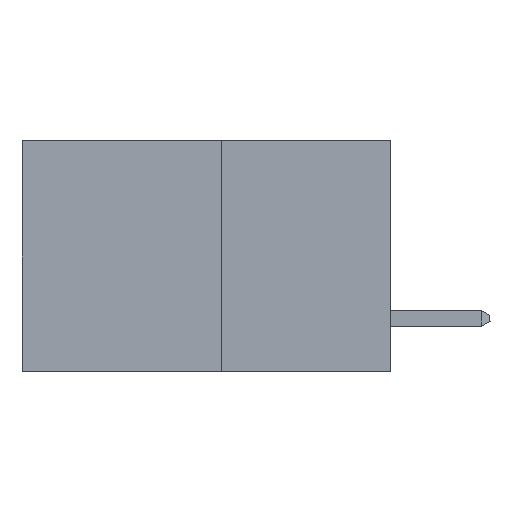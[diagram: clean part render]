
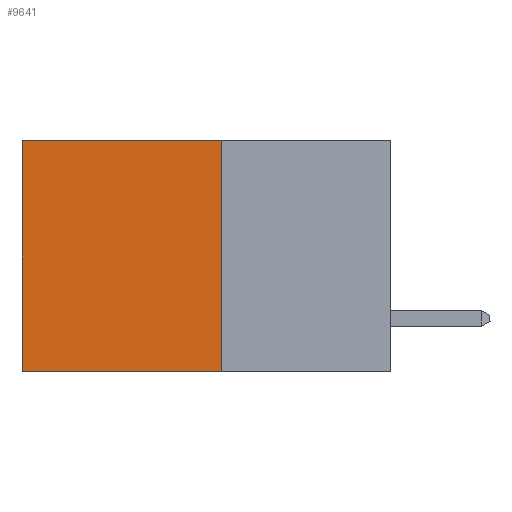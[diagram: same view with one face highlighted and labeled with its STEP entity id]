
A CAD part, left-side view. The second image highlights one B-rep face of the part: STEP entity #9641.
In plain terms, the highlighted planar face has unit normal (-1, 0, 0).
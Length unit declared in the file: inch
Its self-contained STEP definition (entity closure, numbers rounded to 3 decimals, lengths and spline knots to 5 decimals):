
#358 = AXIS2_PLACEMENT_3D ( 'NONE', #10033, #2748, #11231 ) ;
#535 = EDGE_CURVE ( 'NONE', #11754, #8531, #8015, .T. ) ;
#1074 = CARTESIAN_POINT ( 'NONE',  ( 0.277, 0.59, 0. ) ) ;
#1254 = EDGE_CURVE ( 'NONE', #7984, #7675, #7183, .T. ) ;
#1770 = LINE ( 'NONE', #3849, #7908 ) ;
#2586 = DIRECTION ( 'NONE',  ( 0., 1., 0. ) ) ;
#2630 = PLANE ( 'NONE',  #358 ) ;
#2748 = DIRECTION ( 'NONE',  ( 1., 0., 0. ) ) ;
#3657 = ORIENTED_EDGE ( 'NONE', *, *, #9433, .F. ) ;
#3849 = CARTESIAN_POINT ( 'NONE',  ( 0.277, 0.27, 0. ) ) ;
#3951 = VECTOR ( 'NONE', #7203, 39.37008 ) ;
#5088 = VECTOR ( 'NONE', #8420, 39.37008 ) ;
#5573 = ORIENTED_EDGE ( 'NONE', *, *, #535, .F. ) ;
#6667 = CARTESIAN_POINT ( 'NONE',  ( 0.277, 0.27, -0.37 ) ) ;
#7183 = LINE ( 'NONE', #7550, #3951 ) ;
#7203 = DIRECTION ( 'NONE',  ( 0., 0., -1. ) ) ;
#7550 = CARTESIAN_POINT ( 'NONE',  ( 0.277, 0.59, -0.37 ) ) ;
#7675 = VERTEX_POINT ( 'NONE', #9093 ) ;
#7908 = VECTOR ( 'NONE', #2586, 39.37008 ) ;
#7984 = VERTEX_POINT ( 'NONE', #1074 ) ;
#8015 = LINE ( 'NONE', #6667, #13996 ) ;
#8255 = LINE ( 'NONE', #10805, #5088 ) ;
#8387 = CARTESIAN_POINT ( 'NONE',  ( 0.277, 0.27, 0. ) ) ;
#8420 = DIRECTION ( 'NONE',  ( 0., 1., 0. ) ) ;
#8439 = FACE_OUTER_BOUND ( 'NONE', #12865, .T. ) ;
#8531 = VERTEX_POINT ( 'NONE', #12613 ) ;
#9013 = EDGE_CURVE ( 'NONE', #11754, #7984, #1770, .T. ) ;
#9093 = CARTESIAN_POINT ( 'NONE',  ( 0.277, 0.59, -0.37 ) ) ;
#9152 = ORIENTED_EDGE ( 'NONE', *, *, #9013, .T. ) ;
#9433 = EDGE_CURVE ( 'NONE', #8531, #7675, #8255, .T. ) ;
#9641 = ADVANCED_FACE ( 'NONE', ( #8439 ), #2630, .F. ) ;
#10033 = CARTESIAN_POINT ( 'NONE',  ( 0.277, 0.27, -0.37 ) ) ;
#10587 = DIRECTION ( 'NONE',  ( 0., 0., -1. ) ) ;
#10805 = CARTESIAN_POINT ( 'NONE',  ( 0.277, 0.27, -0.37 ) ) ;
#11231 = DIRECTION ( 'NONE',  ( 0., 0., -1. ) ) ;
#11754 = VERTEX_POINT ( 'NONE', #8387 ) ;
#11763 = ORIENTED_EDGE ( 'NONE', *, *, #1254, .T. ) ;
#12613 = CARTESIAN_POINT ( 'NONE',  ( 0.277, 0.27, -0.37 ) ) ;
#12865 = EDGE_LOOP ( 'NONE', ( #11763, #3657, #5573, #9152 ) ) ;
#13996 = VECTOR ( 'NONE', #10587, 39.37008 ) ;
